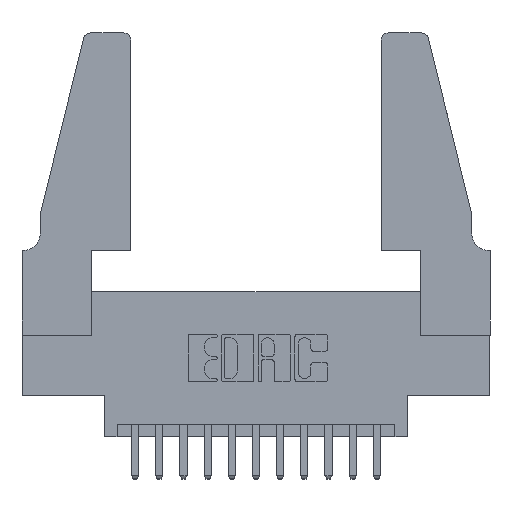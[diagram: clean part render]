
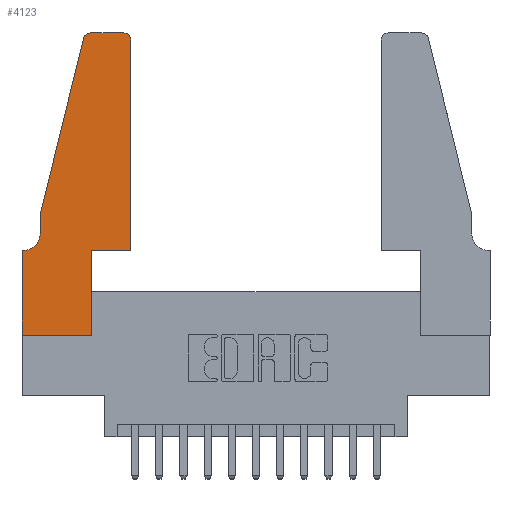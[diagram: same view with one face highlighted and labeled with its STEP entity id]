
A CAD part, top view. The second image highlights one B-rep face of the part: STEP entity #4123.
In plain terms, the highlighted planar face has unit normal (0, 0, 1).
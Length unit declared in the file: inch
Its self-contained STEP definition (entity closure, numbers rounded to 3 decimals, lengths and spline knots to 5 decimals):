
#5 = CARTESIAN_POINT ( 'NONE',  ( 0.0755, 0.5, 0.37 ) ) ;
#62 = LINE ( 'NONE', #6278, #3320 ) ;
#90 = EDGE_LOOP ( 'NONE', ( #308, #7286, #6899, #2258, #12571, #1816, #14539, #1558, #5724, #12982, #1603, #1468 ) ) ;
#242 = CARTESIAN_POINT ( 'NONE',  ( 0., 0.35, 0.37 ) ) ;
#308 = ORIENTED_EDGE ( 'NONE', *, *, #2243, .T. ) ;
#370 = CARTESIAN_POINT ( 'NONE',  ( 0.4505, 0.35, 0.37 ) ) ;
#419 = DIRECTION ( 'NONE',  ( -1., 0., 0. ) ) ;
#635 = DIRECTION ( 'NONE',  ( 0., 1., 0. ) ) ;
#1170 = LINE ( 'NONE', #8149, #3640 ) ;
#1172 = VERTEX_POINT ( 'NONE', #4197 ) ;
#1328 = CARTESIAN_POINT ( 'NONE',  ( 0.4505, 0.35, 0.37 ) ) ;
#1468 = ORIENTED_EDGE ( 'NONE', *, *, #4171, .T. ) ;
#1558 = ORIENTED_EDGE ( 'NONE', *, *, #14524, .T. ) ;
#1603 = ORIENTED_EDGE ( 'NONE', *, *, #11473, .T. ) ;
#1663 = VERTEX_POINT ( 'NONE', #9302 ) ;
#1816 = ORIENTED_EDGE ( 'NONE', *, *, #10262, .T. ) ;
#1875 = EDGE_CURVE ( 'NONE', #1172, #6409, #12281, .T. ) ;
#1904 = DIRECTION ( 'NONE',  ( -1., 0., 0. ) ) ;
#2243 = EDGE_CURVE ( 'NONE', #10377, #1172, #10254, .T. ) ;
#2258 = ORIENTED_EDGE ( 'NONE', *, *, #12929, .T. ) ;
#2496 = CIRCLE ( 'NONE', #13429, 0.03 ) ;
#2544 = DIRECTION ( 'NONE',  ( 1., 0., 0. ) ) ;
#2632 = VERTEX_POINT ( 'NONE', #10886 ) ;
#2662 = LINE ( 'NONE', #5487, #14709 ) ;
#2776 = DIRECTION ( 'NONE',  ( 0., -1., 0. ) ) ;
#2783 = VERTEX_POINT ( 'NONE', #8546 ) ;
#2885 = FACE_OUTER_BOUND ( 'NONE', #90, .T. ) ;
#3320 = VECTOR ( 'NONE', #13201, 39.37008 ) ;
#3640 = VECTOR ( 'NONE', #2776, 39.37008 ) ;
#3719 = VECTOR ( 'NONE', #635, 39.37008 ) ;
#3934 = VERTEX_POINT ( 'NONE', #5094 ) ;
#4071 = EDGE_CURVE ( 'NONE', #8853, #1663, #1170, .T. ) ;
#4123 = ADVANCED_FACE ( 'NONE', ( #2885 ), #15198, .T. ) ;
#4171 = EDGE_CURVE ( 'NONE', #2632, #10377, #2496, .T. ) ;
#4197 = CARTESIAN_POINT ( 'NONE',  ( 0.284, 1.25, 0.37 ) ) ;
#4317 = CARTESIAN_POINT ( 'NONE',  ( 0.0055, 0.42, 0.37 ) ) ;
#4397 = CARTESIAN_POINT ( 'NONE',  ( 0.4205, 1.22, 0.37 ) ) ;
#4504 = CIRCLE ( 'NONE', #15191, 0.07 ) ;
#4879 = VECTOR ( 'NONE', #13099, 39.37008 ) ;
#5040 = DIRECTION ( 'NONE',  ( 1., 0., 0. ) ) ;
#5094 = CARTESIAN_POINT ( 'NONE',  ( 0.0055, 0.35, 0.37 ) ) ;
#5340 = DIRECTION ( 'NONE',  ( -0.239, -0.971, 0. ) ) ;
#5487 = CARTESIAN_POINT ( 'NONE',  ( 0.0755, 0.35, 0.37 ) ) ;
#5519 = DIRECTION ( 'NONE',  ( -1., 0., 0. ) ) ;
#5591 = CARTESIAN_POINT ( 'NONE',  ( 0.0755, 0.42, 0.37 ) ) ;
#5724 = ORIENTED_EDGE ( 'NONE', *, *, #13585, .T. ) ;
#5837 = VECTOR ( 'NONE', #5340, 39.37008 ) ;
#6278 = CARTESIAN_POINT ( 'NONE',  ( 0.0755, 0.5, 0.37 ) ) ;
#6409 = VERTEX_POINT ( 'NONE', #9725 ) ;
#6430 = VERTEX_POINT ( 'NONE', #370 ) ;
#6515 = CARTESIAN_POINT ( 'NONE',  ( 0.2605, 1.25, 0.37 ) ) ;
#6899 = ORIENTED_EDGE ( 'NONE', *, *, #11153, .T. ) ;
#7266 = EDGE_CURVE ( 'NONE', #11853, #3934, #4504, .T. ) ;
#7286 = ORIENTED_EDGE ( 'NONE', *, *, #1875, .T. ) ;
#7312 = DIRECTION ( 'NONE',  ( 0., 0., 1. ) ) ;
#7867 = DIRECTION ( 'NONE',  ( 1., 0., 0. ) ) ;
#7885 = DIRECTION ( 'NONE',  ( 0., 0., 1. ) ) ;
#8149 = CARTESIAN_POINT ( 'NONE',  ( 0., 0., 0.37 ) ) ;
#8166 = EDGE_CURVE ( 'NONE', #2783, #6430, #10604, .T. ) ;
#8509 = CARTESIAN_POINT ( 'NONE',  ( 0., 0., 0.37 ) ) ;
#8546 = CARTESIAN_POINT ( 'NONE',  ( 0.2865, 0.35, 0.37 ) ) ;
#8853 = VERTEX_POINT ( 'NONE', #242 ) ;
#9302 = CARTESIAN_POINT ( 'NONE',  ( 0., 0., 0.37 ) ) ;
#9725 = CARTESIAN_POINT ( 'NONE',  ( 0.25487, 1.22718, 0.37 ) ) ;
#10012 = AXIS2_PLACEMENT_3D ( 'NONE', #14282, #7312, #13988 ) ;
#10237 = LINE ( 'NONE', #8509, #12981 ) ;
#10242 = VECTOR ( 'NONE', #2544, 39.37008 ) ;
#10254 = LINE ( 'NONE', #6515, #13005 ) ;
#10262 = EDGE_CURVE ( 'NONE', #3934, #8853, #2662, .T. ) ;
#10274 = LINE ( 'NONE', #14691, #3719 ) ;
#10377 = VERTEX_POINT ( 'NONE', #14936 ) ;
#10604 = LINE ( 'NONE', #1328, #10242 ) ;
#10626 = DIRECTION ( 'NONE',  ( 0., 0., 1. ) ) ;
#10871 = VERTEX_POINT ( 'NONE', #5 ) ;
#10886 = CARTESIAN_POINT ( 'NONE',  ( 0.4505, 1.22, 0.37 ) ) ;
#11033 = LINE ( 'NONE', #11916, #4879 ) ;
#11146 = CARTESIAN_POINT ( 'NONE',  ( 0.0755, 0.5, 0.37 ) ) ;
#11153 = EDGE_CURVE ( 'NONE', #6409, #10871, #12346, .T. ) ;
#11473 = EDGE_CURVE ( 'NONE', #6430, #2632, #11033, .T. ) ;
#11853 = VERTEX_POINT ( 'NONE', #5591 ) ;
#11916 = CARTESIAN_POINT ( 'NONE',  ( 0.4505, 0.35, 0.37 ) ) ;
#12134 = CARTESIAN_POINT ( 'NONE',  ( 0.2865, 0., 0.37 ) ) ;
#12281 = CIRCLE ( 'NONE', #10012, 0.03 ) ;
#12346 = LINE ( 'NONE', #11146, #5837 ) ;
#12428 = DIRECTION ( 'NONE',  ( 1., 0., 0. ) ) ;
#12465 = DIRECTION ( 'NONE',  ( 0., 0., -1. ) ) ;
#12571 = ORIENTED_EDGE ( 'NONE', *, *, #7266, .T. ) ;
#12667 = AXIS2_PLACEMENT_3D ( 'NONE', #13140, #10626, #12428 ) ;
#12929 = EDGE_CURVE ( 'NONE', #10871, #11853, #62, .T. ) ;
#12969 = VERTEX_POINT ( 'NONE', #12134 ) ;
#12981 = VECTOR ( 'NONE', #5040, 39.37008 ) ;
#12982 = ORIENTED_EDGE ( 'NONE', *, *, #8166, .T. ) ;
#13005 = VECTOR ( 'NONE', #419, 39.37008 ) ;
#13099 = DIRECTION ( 'NONE',  ( 0., 1., 0. ) ) ;
#13140 = CARTESIAN_POINT ( 'NONE',  ( 0., 0.35, 0.37 ) ) ;
#13201 = DIRECTION ( 'NONE',  ( 0., -1., 0. ) ) ;
#13429 = AXIS2_PLACEMENT_3D ( 'NONE', #4397, #7885, #7867 ) ;
#13585 = EDGE_CURVE ( 'NONE', #12969, #2783, #10274, .T. ) ;
#13988 = DIRECTION ( 'NONE',  ( 1., 0., 0. ) ) ;
#14282 = CARTESIAN_POINT ( 'NONE',  ( 0.284, 1.22, 0.37 ) ) ;
#14524 = EDGE_CURVE ( 'NONE', #1663, #12969, #10237, .T. ) ;
#14539 = ORIENTED_EDGE ( 'NONE', *, *, #4071, .T. ) ;
#14691 = CARTESIAN_POINT ( 'NONE',  ( 0.2865, 0.35, 0.37 ) ) ;
#14709 = VECTOR ( 'NONE', #1904, 39.37008 ) ;
#14936 = CARTESIAN_POINT ( 'NONE',  ( 0.4205, 1.25, 0.37 ) ) ;
#15191 = AXIS2_PLACEMENT_3D ( 'NONE', #4317, #12465, #5519 ) ;
#15198 = PLANE ( 'NONE',  #12667 ) ;
